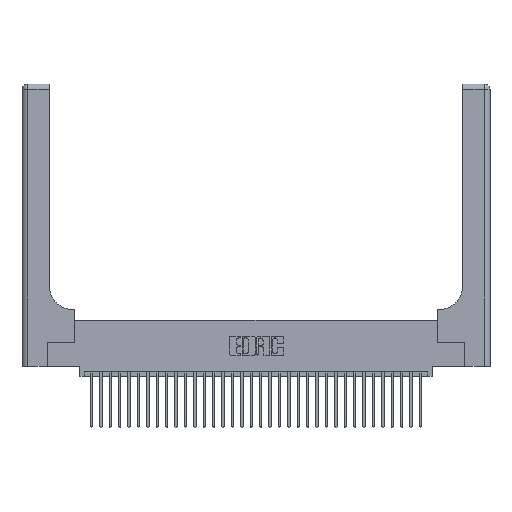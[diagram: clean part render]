
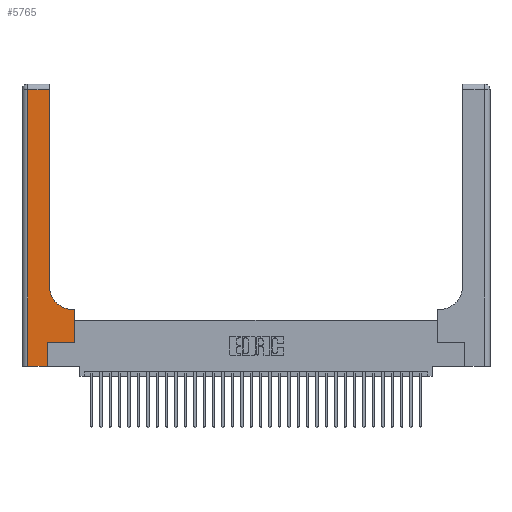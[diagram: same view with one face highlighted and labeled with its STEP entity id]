
A CAD part, top view. The second image highlights one B-rep face of the part: STEP entity #5765.
In plain terms, the highlighted planar face has unit normal (0, 0, 1).
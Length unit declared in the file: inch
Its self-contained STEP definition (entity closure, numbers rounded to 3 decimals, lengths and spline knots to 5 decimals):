
#238 = EDGE_CURVE ( 'NONE', #16081, #7791, #12381, .T. ) ;
#285 = FACE_OUTER_BOUND ( 'NONE', #16561, .T. ) ;
#879 = VERTEX_POINT ( 'NONE', #24347 ) ;
#1168 = DIRECTION ( 'NONE',  ( 0., 0., -1. ) ) ;
#1462 = CARTESIAN_POINT ( 'NONE',  ( 0.5415, 0.6, 0.37 ) ) ;
#2117 = ORIENTED_EDGE ( 'NONE', *, *, #16661, .T. ) ;
#2536 = CARTESIAN_POINT ( 'NONE',  ( 0.5585, 0.6, 0.37 ) ) ;
#2702 = VERTEX_POINT ( 'NONE', #12582 ) ;
#3605 = CARTESIAN_POINT ( 'NONE',  ( 0.2915, 0.6, 0.37 ) ) ;
#4419 = EDGE_CURVE ( 'NONE', #21629, #14193, #27427, .T. ) ;
#4610 = EDGE_CURVE ( 'NONE', #8488, #18710, #14123, .T. ) ;
#5062 = EDGE_CURVE ( 'NONE', #14193, #16081, #20424, .T. ) ;
#5108 = LINE ( 'NONE', #3605, #11384 ) ;
#5765 = ADVANCED_FACE ( 'NONE', ( #285 ), #32996, .F. ) ;
#5845 = DIRECTION ( 'NONE',  ( 1., 0., 0. ) ) ;
#6164 = VECTOR ( 'NONE', #32923, 39.37008 ) ;
#6400 = CARTESIAN_POINT ( 'NONE',  ( 0., 3., 0.37 ) ) ;
#6707 = CARTESIAN_POINT ( 'NONE',  ( 0.269, 0., 0.37 ) ) ;
#7791 = VERTEX_POINT ( 'NONE', #6707 ) ;
#7965 = ORIENTED_EDGE ( 'NONE', *, *, #238, .T. ) ;
#8277 = EDGE_CURVE ( 'NONE', #879, #8488, #15962, .T. ) ;
#8410 = ORIENTED_EDGE ( 'NONE', *, *, #8277, .T. ) ;
#8488 = VERTEX_POINT ( 'NONE', #25516 ) ;
#8795 = ORIENTED_EDGE ( 'NONE', *, *, #26461, .T. ) ;
#8858 = CIRCLE ( 'NONE', #14093, 0.25 ) ;
#9463 = CARTESIAN_POINT ( 'NONE',  ( 0.2915, 3., 0.37 ) ) ;
#9891 = VECTOR ( 'NONE', #14835, 39.37008 ) ;
#11384 = VECTOR ( 'NONE', #11764, 39.37008 ) ;
#11764 = DIRECTION ( 'NONE',  ( -1., 0., 0. ) ) ;
#12381 = LINE ( 'NONE', #31858, #25731 ) ;
#12450 = CARTESIAN_POINT ( 'NONE',  ( 0.5415, 0.85, 0.37 ) ) ;
#12582 = CARTESIAN_POINT ( 'NONE',  ( 0.2915, 0.85, 0.37 ) ) ;
#13273 = LINE ( 'NONE', #31504, #33627 ) ;
#14093 = AXIS2_PLACEMENT_3D ( 'NONE', #12450, #31048, #15149 ) ;
#14123 = LINE ( 'NONE', #30918, #27466 ) ;
#14193 = VERTEX_POINT ( 'NONE', #28308 ) ;
#14416 = CARTESIAN_POINT ( 'NONE',  ( 0., 2.94, 0.37 ) ) ;
#14835 = DIRECTION ( 'NONE',  ( 0., 1., 0. ) ) ;
#15120 = VECTOR ( 'NONE', #5845, 39.37008 ) ;
#15149 = DIRECTION ( 'NONE',  ( 1., 0., 0. ) ) ;
#15962 = LINE ( 'NONE', #24363, #15120 ) ;
#16081 = VERTEX_POINT ( 'NONE', #19945 ) ;
#16561 = EDGE_LOOP ( 'NONE', ( #2117, #17144, #18852, #7965, #8795, #8410, #22620, #24244, #25925 ) ) ;
#16661 = EDGE_CURVE ( 'NONE', #2702, #21629, #24063, .T. ) ;
#17106 = DIRECTION ( 'NONE',  ( -1., 0., 0. ) ) ;
#17144 = ORIENTED_EDGE ( 'NONE', *, *, #4419, .T. ) ;
#18710 = VERTEX_POINT ( 'NONE', #2536 ) ;
#18852 = ORIENTED_EDGE ( 'NONE', *, *, #5062, .T. ) ;
#19431 = AXIS2_PLACEMENT_3D ( 'NONE', #6400, #1168, #19865 ) ;
#19788 = CARTESIAN_POINT ( 'NONE',  ( 0.06, 3., 0.37 ) ) ;
#19865 = DIRECTION ( 'NONE',  ( -1., 0., 0. ) ) ;
#19945 = CARTESIAN_POINT ( 'NONE',  ( 0.06, 0., 0.37 ) ) ;
#20424 = LINE ( 'NONE', #19788, #6164 ) ;
#21345 = VERTEX_POINT ( 'NONE', #1462 ) ;
#21629 = VERTEX_POINT ( 'NONE', #26575 ) ;
#22620 = ORIENTED_EDGE ( 'NONE', *, *, #4610, .T. ) ;
#24063 = LINE ( 'NONE', #9463, #9891 ) ;
#24244 = ORIENTED_EDGE ( 'NONE', *, *, #30558, .T. ) ;
#24347 = CARTESIAN_POINT ( 'NONE',  ( 0.269, 0.25, 0.37 ) ) ;
#24363 = CARTESIAN_POINT ( 'NONE',  ( 0.269, 0.25, 0.37 ) ) ;
#25516 = CARTESIAN_POINT ( 'NONE',  ( 0.5585, 0.25, 0.37 ) ) ;
#25731 = VECTOR ( 'NONE', #31558, 39.37008 ) ;
#25766 = VECTOR ( 'NONE', #17106, 39.37008 ) ;
#25925 = ORIENTED_EDGE ( 'NONE', *, *, #30706, .T. ) ;
#26461 = EDGE_CURVE ( 'NONE', #7791, #879, #13273, .T. ) ;
#26575 = CARTESIAN_POINT ( 'NONE',  ( 0.2915, 2.94, 0.37 ) ) ;
#27427 = LINE ( 'NONE', #14416, #25766 ) ;
#27466 = VECTOR ( 'NONE', #28393, 39.37008 ) ;
#28308 = CARTESIAN_POINT ( 'NONE',  ( 0.06, 2.94, 0.37 ) ) ;
#28393 = DIRECTION ( 'NONE',  ( 0., 1., 0. ) ) ;
#28876 = DIRECTION ( 'NONE',  ( 0., 1., 0. ) ) ;
#30558 = EDGE_CURVE ( 'NONE', #18710, #21345, #5108, .T. ) ;
#30706 = EDGE_CURVE ( 'NONE', #21345, #2702, #8858, .T. ) ;
#30918 = CARTESIAN_POINT ( 'NONE',  ( 0.5585, 0.25, 0.37 ) ) ;
#31048 = DIRECTION ( 'NONE',  ( 0., 0., -1. ) ) ;
#31504 = CARTESIAN_POINT ( 'NONE',  ( 0.269, 0., 0.37 ) ) ;
#31558 = DIRECTION ( 'NONE',  ( 1., 0., 0. ) ) ;
#31858 = CARTESIAN_POINT ( 'NONE',  ( 0., 0., 0.37 ) ) ;
#32923 = DIRECTION ( 'NONE',  ( 0., -1., 0. ) ) ;
#32996 = PLANE ( 'NONE',  #19431 ) ;
#33627 = VECTOR ( 'NONE', #28876, 39.37008 ) ;
